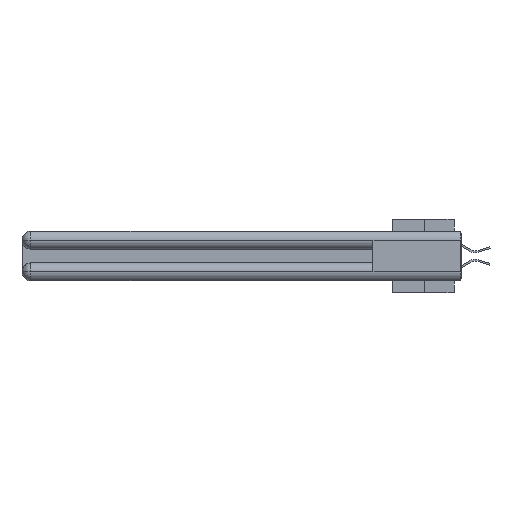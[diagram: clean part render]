
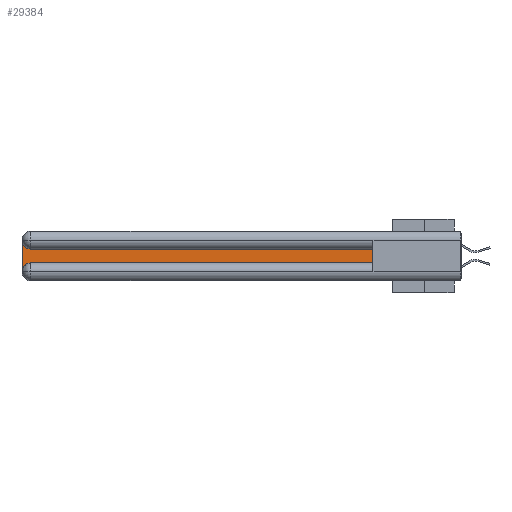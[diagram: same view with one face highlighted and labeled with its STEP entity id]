
A CAD part, left-side view. The second image highlights one B-rep face of the part: STEP entity #29384.
In plain terms, the highlighted planar face has unit normal (-1, 0, 0).
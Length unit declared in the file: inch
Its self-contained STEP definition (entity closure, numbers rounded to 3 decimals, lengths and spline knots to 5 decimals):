
#20 = VERTEX_POINT ( 'NONE', #7612 ) ;
#104 = DIRECTION ( 'NONE',  ( 1., 0., 0. ) ) ;
#644 = AXIS2_PLACEMENT_3D ( 'NONE', #11707, #104, #16386 ) ;
#2048 = ORIENTED_EDGE ( 'NONE', *, *, #12065, .T. ) ;
#2799 = DIRECTION ( 'NONE',  ( 0., -1., 0. ) ) ;
#3211 = CIRCLE ( 'NONE', #17853, 0.06 ) ;
#3480 = EDGE_CURVE ( 'NONE', #29022, #13333, #10846, .T. ) ;
#3509 = ORIENTED_EDGE ( 'NONE', *, *, #3480, .T. ) ;
#4580 = CIRCLE ( 'NONE', #11762, 0.06 ) ;
#6049 = DIRECTION ( 'NONE',  ( 0., 1., 0. ) ) ;
#6516 = VERTEX_POINT ( 'NONE', #19496 ) ;
#7612 = CARTESIAN_POINT ( 'NONE',  ( 0.075, 0.6, -0.1225 ) ) ;
#8230 = DIRECTION ( 'NONE',  ( 0., 0., 1. ) ) ;
#9131 = ORIENTED_EDGE ( 'NONE', *, *, #29060, .T. ) ;
#10846 = LINE ( 'NONE', #28884, #13409 ) ;
#10938 = CARTESIAN_POINT ( 'NONE',  ( 0.075, 2.94, -0.0625 ) ) ;
#11138 = LINE ( 'NONE', #26996, #28942 ) ;
#11707 = CARTESIAN_POINT ( 'NONE',  ( 0.075, 3., -0.1225 ) ) ;
#11762 = AXIS2_PLACEMENT_3D ( 'NONE', #13441, #22647, #29488 ) ;
#12065 = EDGE_CURVE ( 'NONE', #12395, #6516, #23608, .T. ) ;
#12304 = EDGE_CURVE ( 'NONE', #20886, #29022, #3211, .T. ) ;
#12395 = VERTEX_POINT ( 'NONE', #20182 ) ;
#13333 = VERTEX_POINT ( 'NONE', #20382 ) ;
#13409 = VECTOR ( 'NONE', #20041, 39.37008 ) ;
#13441 = CARTESIAN_POINT ( 'NONE',  ( 0.075, 2.94, -0.2775 ) ) ;
#14737 = ORIENTED_EDGE ( 'NONE', *, *, #26172, .T. ) ;
#16386 = DIRECTION ( 'NONE',  ( 0., 0., -1. ) ) ;
#16702 = LINE ( 'NONE', #27156, #29825 ) ;
#17853 = AXIS2_PLACEMENT_3D ( 'NONE', #10938, #24782, #22305 ) ;
#18842 = EDGE_LOOP ( 'NONE', ( #9131, #22051, #3509, #24579, #2048, #14737 ) ) ;
#19130 = FACE_OUTER_BOUND ( 'NONE', #18842, .T. ) ;
#19496 = CARTESIAN_POINT ( 'NONE',  ( 0.075, 0.6, -0.2175 ) ) ;
#20041 = DIRECTION ( 'NONE',  ( 0., 0., -1. ) ) ;
#20182 = CARTESIAN_POINT ( 'NONE',  ( 0.075, 2.94, -0.2175 ) ) ;
#20382 = CARTESIAN_POINT ( 'NONE',  ( 0.075, 3., -0.2775 ) ) ;
#20886 = VERTEX_POINT ( 'NONE', #29787 ) ;
#22051 = ORIENTED_EDGE ( 'NONE', *, *, #12304, .T. ) ;
#22305 = DIRECTION ( 'NONE',  ( 0., 0., -1. ) ) ;
#22540 = EDGE_CURVE ( 'NONE', #13333, #12395, #4580, .T. ) ;
#22647 = DIRECTION ( 'NONE',  ( 1., 0., 0. ) ) ;
#23300 = PLANE ( 'NONE',  #644 ) ;
#23608 = LINE ( 'NONE', #27737, #29068 ) ;
#24579 = ORIENTED_EDGE ( 'NONE', *, *, #22540, .T. ) ;
#24782 = DIRECTION ( 'NONE',  ( 1., 0., 0. ) ) ;
#26172 = EDGE_CURVE ( 'NONE', #6516, #20, #16702, .T. ) ;
#26890 = CARTESIAN_POINT ( 'NONE',  ( 0.075, 3., -0.0625 ) ) ;
#26996 = CARTESIAN_POINT ( 'NONE',  ( 0.075, 0.6, -0.1225 ) ) ;
#27156 = CARTESIAN_POINT ( 'NONE',  ( 0.075, 0.6, -0.2175 ) ) ;
#27737 = CARTESIAN_POINT ( 'NONE',  ( 0.075, 0.6, -0.2175 ) ) ;
#28884 = CARTESIAN_POINT ( 'NONE',  ( 0.075, 3., -0.2175 ) ) ;
#28942 = VECTOR ( 'NONE', #6049, 39.37008 ) ;
#29022 = VERTEX_POINT ( 'NONE', #26890 ) ;
#29060 = EDGE_CURVE ( 'NONE', #20, #20886, #11138, .T. ) ;
#29068 = VECTOR ( 'NONE', #2799, 39.37008 ) ;
#29384 = ADVANCED_FACE ( 'NONE', ( #19130 ), #23300, .F. ) ;
#29488 = DIRECTION ( 'NONE',  ( 0., 0., -1. ) ) ;
#29787 = CARTESIAN_POINT ( 'NONE',  ( 0.075, 2.94, -0.1225 ) ) ;
#29825 = VECTOR ( 'NONE', #8230, 39.37008 ) ;
